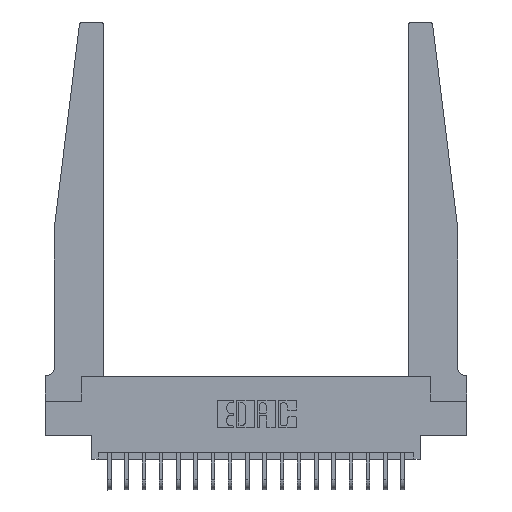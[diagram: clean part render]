
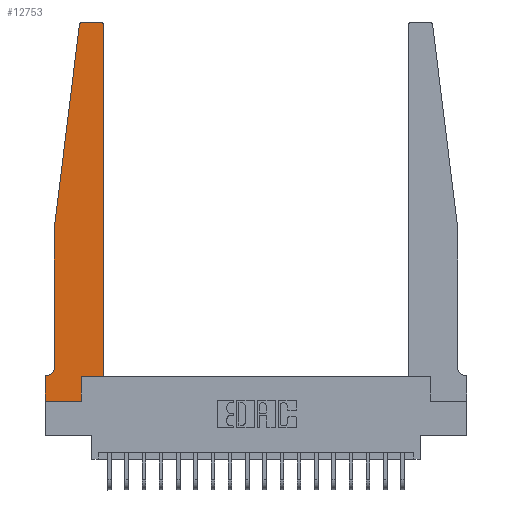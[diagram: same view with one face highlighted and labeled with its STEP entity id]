
A CAD part, top view. The second image highlights one B-rep face of the part: STEP entity #12753.
In plain terms, the highlighted planar face has unit normal (0, 0, 1).
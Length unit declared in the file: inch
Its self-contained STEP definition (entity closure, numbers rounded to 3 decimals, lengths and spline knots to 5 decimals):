
#14 = VERTEX_POINT ( 'NONE', #7662 ) ;
#42 = EDGE_CURVE ( 'NONE', #2163, #11438, #12456, .T. ) ;
#438 = CARTESIAN_POINT ( 'NONE',  ( 0.425, 2.72, 0.37 ) ) ;
#510 = VERTEX_POINT ( 'NONE', #14019 ) ;
#643 = CARTESIAN_POINT ( 'NONE',  ( 0.395, 2.75, 0.37 ) ) ;
#667 = CARTESIAN_POINT ( 'NONE',  ( 0.015, 0.2375, 0.37 ) ) ;
#721 = VECTOR ( 'NONE', #16714, 39.37008 ) ;
#1162 = DIRECTION ( 'NONE',  ( 1., 0., 0. ) ) ;
#1260 = LINE ( 'NONE', #8107, #17365 ) ;
#2163 = VERTEX_POINT ( 'NONE', #438 ) ;
#2223 = VECTOR ( 'NONE', #4579, 39.37008 ) ;
#2604 = VERTEX_POINT ( 'NONE', #3659 ) ;
#2814 = CARTESIAN_POINT ( 'NONE',  ( 0., 0., 0.37 ) ) ;
#2836 = CARTESIAN_POINT ( 'NONE',  ( 0.24675, 2.72367, 0.37 ) ) ;
#2844 = VERTEX_POINT ( 'NONE', #17714 ) ;
#2943 = VECTOR ( 'NONE', #15497, 39.37008 ) ;
#2972 = VERTEX_POINT ( 'NONE', #18934 ) ;
#3028 = ORIENTED_EDGE ( 'NONE', *, *, #18645, .T. ) ;
#3046 = PLANE ( 'NONE',  #14702 ) ;
#3472 = ORIENTED_EDGE ( 'NONE', *, *, #8188, .T. ) ;
#3586 = ORIENTED_EDGE ( 'NONE', *, *, #10506, .T. ) ;
#3659 = CARTESIAN_POINT ( 'NONE',  ( 0.065, 0.2375, 0.37 ) ) ;
#3697 = ORIENTED_EDGE ( 'NONE', *, *, #7255, .T. ) ;
#4579 = DIRECTION ( 'NONE',  ( 1., 0., 0. ) ) ;
#4723 = DIRECTION ( 'NONE',  ( -1., 0., 0. ) ) ;
#5118 = ORIENTED_EDGE ( 'NONE', *, *, #7038, .T. ) ;
#5322 = DIRECTION ( 'NONE',  ( 1., 0., 0. ) ) ;
#5817 = DIRECTION ( 'NONE',  ( -1., 0., 0. ) ) ;
#5983 = VECTOR ( 'NONE', #5322, 39.37008 ) ;
#6158 = AXIS2_PLACEMENT_3D ( 'NONE', #667, #7510, #5817 ) ;
#6221 = ORIENTED_EDGE ( 'NONE', *, *, #8635, .T. ) ;
#6361 = DIRECTION ( 'NONE',  ( 1., 0., 0. ) ) ;
#6410 = ORIENTED_EDGE ( 'NONE', *, *, #12794, .T. ) ;
#6696 = CARTESIAN_POINT ( 'NONE',  ( 0.27653, 2.72, 0.37 ) ) ;
#6813 = VECTOR ( 'NONE', #17981, 39.37008 ) ;
#6947 = LINE ( 'NONE', #7057, #2943 ) ;
#7038 = EDGE_CURVE ( 'NONE', #2844, #13580, #18100, .T. ) ;
#7057 = CARTESIAN_POINT ( 'NONE',  ( 0.2605, 0.18, 0.37 ) ) ;
#7255 = EDGE_CURVE ( 'NONE', #11438, #18230, #21752, .T. ) ;
#7510 = DIRECTION ( 'NONE',  ( 0., 0., -1. ) ) ;
#7662 = CARTESIAN_POINT ( 'NONE',  ( 0.425, 0.18, 0.37 ) ) ;
#7724 = LINE ( 'NONE', #19690, #16914 ) ;
#7773 = DIRECTION ( 'NONE',  ( -0.122, -0.992, 0. ) ) ;
#7954 = FACE_OUTER_BOUND ( 'NONE', #14436, .T. ) ;
#8107 = CARTESIAN_POINT ( 'NONE',  ( 0.065, 1.25, 0.37 ) ) ;
#8188 = EDGE_CURVE ( 'NONE', #2972, #19970, #6947, .T. ) ;
#8349 = CARTESIAN_POINT ( 'NONE',  ( 0., 0., 0.37 ) ) ;
#8457 = CARTESIAN_POINT ( 'NONE',  ( 0.425, 0.18, 0.37 ) ) ;
#8635 = EDGE_CURVE ( 'NONE', #13580, #2972, #16608, .T. ) ;
#8709 = ORIENTED_EDGE ( 'NONE', *, *, #42, .T. ) ;
#8771 = CARTESIAN_POINT ( 'NONE',  ( 0.065, 1.25, 0.37 ) ) ;
#9175 = AXIS2_PLACEMENT_3D ( 'NONE', #6696, #21050, #10242 ) ;
#9581 = CARTESIAN_POINT ( 'NONE',  ( 0.27653, 2.75, 0.37 ) ) ;
#9699 = ORIENTED_EDGE ( 'NONE', *, *, #21432, .T. ) ;
#9913 = ORIENTED_EDGE ( 'NONE', *, *, #20589, .T. ) ;
#10223 = CARTESIAN_POINT ( 'NONE',  ( 0.425, 0.18, 0.37 ) ) ;
#10242 = DIRECTION ( 'NONE',  ( 1., 0., 0. ) ) ;
#10475 = CARTESIAN_POINT ( 'NONE',  ( 0.065, 1.25, 0.37 ) ) ;
#10506 = EDGE_CURVE ( 'NONE', #10621, #2604, #19209, .T. ) ;
#10621 = VERTEX_POINT ( 'NONE', #8771 ) ;
#11383 = EDGE_CURVE ( 'NONE', #2604, #510, #15393, .T. ) ;
#11438 = VERTEX_POINT ( 'NONE', #643 ) ;
#12135 = DIRECTION ( 'NONE',  ( 0., -1., 0. ) ) ;
#12456 = CIRCLE ( 'NONE', #21402, 0.03 ) ;
#12753 = ADVANCED_FACE ( 'NONE', ( #7954 ), #3046, .T. ) ;
#12794 = EDGE_CURVE ( 'NONE', #510, #2844, #7724, .T. ) ;
#13244 = CARTESIAN_POINT ( 'NONE',  ( 0.25, 2.75, 0.37 ) ) ;
#13354 = ORIENTED_EDGE ( 'NONE', *, *, #11383, .T. ) ;
#13580 = VERTEX_POINT ( 'NONE', #8349 ) ;
#14019 = CARTESIAN_POINT ( 'NONE',  ( 0.015, 0.1875, 0.37 ) ) ;
#14436 = EDGE_LOOP ( 'NONE', ( #3697, #9699, #3028, #3586, #13354, #6410, #5118, #6221, #3472, #19037, #9913, #8709 ) ) ;
#14702 = AXIS2_PLACEMENT_3D ( 'NONE', #19800, #16298, #6361 ) ;
#15210 = DIRECTION ( 'NONE',  ( 0., 1., 0. ) ) ;
#15393 = CIRCLE ( 'NONE', #6158, 0.05 ) ;
#15497 = DIRECTION ( 'NONE',  ( 0., 1., 0. ) ) ;
#16298 = DIRECTION ( 'NONE',  ( 0., 0., 1. ) ) ;
#16608 = LINE ( 'NONE', #18194, #2223 ) ;
#16714 = DIRECTION ( 'NONE',  ( -1., 0., 0. ) ) ;
#16914 = VECTOR ( 'NONE', #4723, 39.37008 ) ;
#17023 = VECTOR ( 'NONE', #15210, 39.37008 ) ;
#17365 = VECTOR ( 'NONE', #7773, 39.37008 ) ;
#17371 = LINE ( 'NONE', #10223, #5983 ) ;
#17714 = CARTESIAN_POINT ( 'NONE',  ( 0., 0.1875, 0.37 ) ) ;
#17931 = DIRECTION ( 'NONE',  ( 0., 0., 1. ) ) ;
#17981 = DIRECTION ( 'NONE',  ( 0., -1., 0. ) ) ;
#18100 = LINE ( 'NONE', #2814, #6813 ) ;
#18168 = CARTESIAN_POINT ( 'NONE',  ( 0.395, 2.72, 0.37 ) ) ;
#18194 = CARTESIAN_POINT ( 'NONE',  ( 0., 0., 0.37 ) ) ;
#18230 = VERTEX_POINT ( 'NONE', #9581 ) ;
#18645 = EDGE_CURVE ( 'NONE', #20835, #10621, #1260, .T. ) ;
#18814 = CIRCLE ( 'NONE', #9175, 0.03 ) ;
#18934 = CARTESIAN_POINT ( 'NONE',  ( 0.2605, 0., 0.37 ) ) ;
#19037 = ORIENTED_EDGE ( 'NONE', *, *, #19741, .T. ) ;
#19209 = LINE ( 'NONE', #10475, #20424 ) ;
#19690 = CARTESIAN_POINT ( 'NONE',  ( 0.065, 0.1875, 0.37 ) ) ;
#19741 = EDGE_CURVE ( 'NONE', #19970, #14, #17371, .T. ) ;
#19800 = CARTESIAN_POINT ( 'NONE',  ( 0., 0.1875, 0.37 ) ) ;
#19955 = CARTESIAN_POINT ( 'NONE',  ( 0.2605, 0.18, 0.37 ) ) ;
#19970 = VERTEX_POINT ( 'NONE', #19955 ) ;
#20096 = LINE ( 'NONE', #8457, #17023 ) ;
#20424 = VECTOR ( 'NONE', #12135, 39.37008 ) ;
#20589 = EDGE_CURVE ( 'NONE', #14, #2163, #20096, .T. ) ;
#20835 = VERTEX_POINT ( 'NONE', #2836 ) ;
#21050 = DIRECTION ( 'NONE',  ( 0., 0., 1. ) ) ;
#21402 = AXIS2_PLACEMENT_3D ( 'NONE', #18168, #17931, #1162 ) ;
#21432 = EDGE_CURVE ( 'NONE', #18230, #20835, #18814, .T. ) ;
#21752 = LINE ( 'NONE', #13244, #721 ) ;
